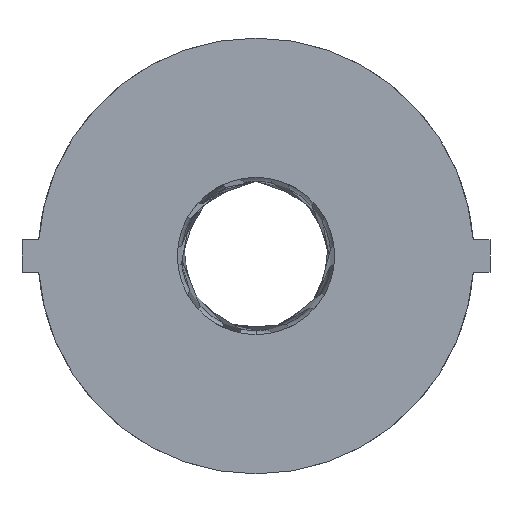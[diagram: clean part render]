
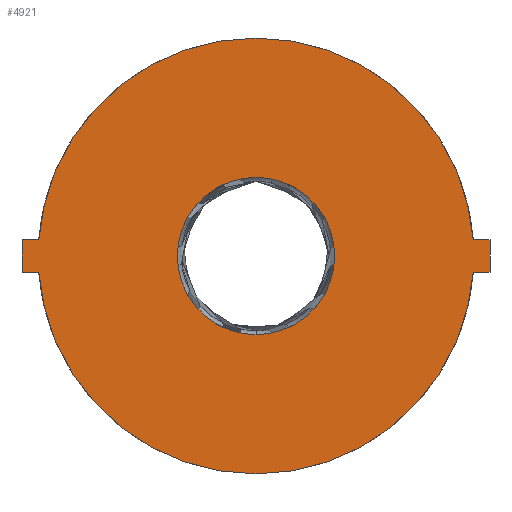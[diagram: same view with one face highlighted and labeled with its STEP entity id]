
A CAD part, front view. The second image highlights one B-rep face of the part: STEP entity #4921.
In plain terms, the highlighted planar face has unit normal (0, -1, 0).
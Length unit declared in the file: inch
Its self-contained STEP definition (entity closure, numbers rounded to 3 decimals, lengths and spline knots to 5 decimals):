
#85 = EDGE_CURVE ( 'NONE', #1512, #594, #125, .T. ) ;
#125 = CIRCLE ( 'NONE', #4471, 0.54 ) ;
#191 = ORIENTED_EDGE ( 'NONE', *, *, #5445, .T. ) ;
#195 = LINE ( 'NONE', #5136, #3071 ) ;
#203 = EDGE_CURVE ( 'NONE', #1984, #433, #4160, .T. ) ;
#219 = VECTOR ( 'NONE', #4748, 39.37008 ) ;
#260 = VERTEX_POINT ( 'NONE', #291 ) ;
#291 = CARTESIAN_POINT ( 'NONE',  ( -0.58, 0., 0.04 ) ) ;
#392 = EDGE_LOOP ( 'NONE', ( #191, #1604 ) ) ;
#433 = VERTEX_POINT ( 'NONE', #6482 ) ;
#450 = DIRECTION ( 'NONE',  ( 1., 0., 0. ) ) ;
#456 = VECTOR ( 'NONE', #450, 39.37008 ) ;
#557 = CARTESIAN_POINT ( 'NONE',  ( -0.58, 0., -0.04 ) ) ;
#594 = VERTEX_POINT ( 'NONE', #6602 ) ;
#601 = CARTESIAN_POINT ( 'NONE',  ( 0., 0., 0.54 ) ) ;
#624 = CIRCLE ( 'NONE', #6725, 0.54 ) ;
#656 = CARTESIAN_POINT ( 'NONE',  ( 0.58, 0., 0.04 ) ) ;
#1033 = ORIENTED_EDGE ( 'NONE', *, *, #3406, .T. ) ;
#1054 = CARTESIAN_POINT ( 'NONE',  ( 0., 0., 0. ) ) ;
#1084 = DIRECTION ( 'NONE',  ( -1., 0., 0. ) ) ;
#1099 = VERTEX_POINT ( 'NONE', #1756 ) ;
#1248 = DIRECTION ( 'NONE',  ( 0., 0., 1. ) ) ;
#1254 = EDGE_CURVE ( 'NONE', #4690, #3625, #2750, .T. ) ;
#1309 = CIRCLE ( 'NONE', #4706, 0.195 ) ;
#1450 = AXIS2_PLACEMENT_3D ( 'NONE', #6536, #3787, #6466 ) ;
#1512 = VERTEX_POINT ( 'NONE', #2586 ) ;
#1524 = CARTESIAN_POINT ( 'NONE',  ( 0., 0., 0.04 ) ) ;
#1604 = ORIENTED_EDGE ( 'NONE', *, *, #3862, .T. ) ;
#1605 = CARTESIAN_POINT ( 'NONE',  ( -0.58, 0., 0. ) ) ;
#1655 = CIRCLE ( 'NONE', #5702, 0.54 ) ;
#1756 = CARTESIAN_POINT ( 'NONE',  ( 0., 0., -0.195 ) ) ;
#1763 = CARTESIAN_POINT ( 'NONE',  ( -0.53852, 0., 0.04 ) ) ;
#1826 = CIRCLE ( 'NONE', #5029, 0.195 ) ;
#1984 = VERTEX_POINT ( 'NONE', #2111 ) ;
#1992 = FACE_BOUND ( 'NONE', #392, .T. ) ;
#2099 = EDGE_CURVE ( 'NONE', #433, #1512, #1655, .T. ) ;
#2111 = CARTESIAN_POINT ( 'NONE',  ( 0.58, 0., -0.04 ) ) ;
#2150 = AXIS2_PLACEMENT_3D ( 'NONE', #4991, #6590, #3428 ) ;
#2356 = ORIENTED_EDGE ( 'NONE', *, *, #6309, .T. ) ;
#2586 = CARTESIAN_POINT ( 'NONE',  ( 0., 0., -0.54 ) ) ;
#2596 = CARTESIAN_POINT ( 'NONE',  ( 0., 0., -0.04 ) ) ;
#2605 = ORIENTED_EDGE ( 'NONE', *, *, #203, .F. ) ;
#2703 = CARTESIAN_POINT ( 'NONE',  ( 0., 0., 0. ) ) ;
#2714 = VERTEX_POINT ( 'NONE', #557 ) ;
#2750 = CIRCLE ( 'NONE', #1450, 0.54 ) ;
#2804 = EDGE_CURVE ( 'NONE', #4629, #3024, #3236, .T. ) ;
#2854 = PLANE ( 'NONE',  #2150 ) ;
#3017 = ORIENTED_EDGE ( 'NONE', *, *, #2099, .F. ) ;
#3024 = VERTEX_POINT ( 'NONE', #3293 ) ;
#3071 = VECTOR ( 'NONE', #5674, 39.37008 ) ;
#3195 = ORIENTED_EDGE ( 'NONE', *, *, #4025, .F. ) ;
#3236 = LINE ( 'NONE', #5679, #4230 ) ;
#3293 = CARTESIAN_POINT ( 'NONE',  ( 0.53852, 0., 0.04 ) ) ;
#3406 = EDGE_CURVE ( 'NONE', #2714, #594, #5418, .T. ) ;
#3428 = DIRECTION ( 'NONE',  ( 0., 0., 1. ) ) ;
#3493 = DIRECTION ( 'NONE',  ( 0., 0., -1. ) ) ;
#3625 = VERTEX_POINT ( 'NONE', #601 ) ;
#3761 = DIRECTION ( 'NONE',  ( 0., 0., 1. ) ) ;
#3787 = DIRECTION ( 'NONE',  ( 0., 1., 0. ) ) ;
#3862 = EDGE_CURVE ( 'NONE', #6628, #1099, #1309, .T. ) ;
#3936 = EDGE_LOOP ( 'NONE', ( #3017, #2605, #5635, #4362, #3195, #4037, #6709, #2356, #1033, #6298 ) ) ;
#3948 = DIRECTION ( 'NONE',  ( 0., 1., 0. ) ) ;
#4025 = EDGE_CURVE ( 'NONE', #3625, #3024, #624, .T. ) ;
#4037 = ORIENTED_EDGE ( 'NONE', *, *, #1254, .F. ) ;
#4153 = FACE_OUTER_BOUND ( 'NONE', #3936, .T. ) ;
#4160 = LINE ( 'NONE', #2596, #219 ) ;
#4230 = VECTOR ( 'NONE', #1084, 39.37008 ) ;
#4264 = CARTESIAN_POINT ( 'NONE',  ( 0., 0., 0.195 ) ) ;
#4278 = CARTESIAN_POINT ( 'NONE',  ( 0., 0., 0. ) ) ;
#4303 = DIRECTION ( 'NONE',  ( 1., 0., 0. ) ) ;
#4362 = ORIENTED_EDGE ( 'NONE', *, *, #2804, .T. ) ;
#4381 = EDGE_CURVE ( 'NONE', #1984, #4629, #195, .T. ) ;
#4471 = AXIS2_PLACEMENT_3D ( 'NONE', #4278, #6336, #6893 ) ;
#4480 = DIRECTION ( 'NONE',  ( 0., 0., 1. ) ) ;
#4506 = CARTESIAN_POINT ( 'NONE',  ( 0., 0., 0. ) ) ;
#4629 = VERTEX_POINT ( 'NONE', #656 ) ;
#4690 = VERTEX_POINT ( 'NONE', #1763 ) ;
#4706 = AXIS2_PLACEMENT_3D ( 'NONE', #5340, #4844, #3761 ) ;
#4730 = VECTOR ( 'NONE', #4303, 39.37008 ) ;
#4748 = DIRECTION ( 'NONE',  ( -1., 0., 0. ) ) ;
#4844 = DIRECTION ( 'NONE',  ( 0., 1., 0. ) ) ;
#4852 = CARTESIAN_POINT ( 'NONE',  ( 0., 0., -0.04 ) ) ;
#4921 = ADVANCED_FACE ( 'NONE', ( #4153, #1992 ), #2854, .F. ) ;
#4991 = CARTESIAN_POINT ( 'NONE',  ( 0., 0., 0. ) ) ;
#5029 = AXIS2_PLACEMENT_3D ( 'NONE', #4506, #3948, #4480 ) ;
#5136 = CARTESIAN_POINT ( 'NONE',  ( 0.58, 0., 0. ) ) ;
#5340 = CARTESIAN_POINT ( 'NONE',  ( 0., 0., 0. ) ) ;
#5407 = DIRECTION ( 'NONE',  ( 0., 0., 1. ) ) ;
#5418 = LINE ( 'NONE', #4852, #4730 ) ;
#5445 = EDGE_CURVE ( 'NONE', #1099, #6628, #1826, .T. ) ;
#5534 = EDGE_CURVE ( 'NONE', #260, #4690, #6323, .T. ) ;
#5635 = ORIENTED_EDGE ( 'NONE', *, *, #4381, .T. ) ;
#5674 = DIRECTION ( 'NONE',  ( 0., 0., 1. ) ) ;
#5679 = CARTESIAN_POINT ( 'NONE',  ( 0., 0., 0.04 ) ) ;
#5702 = AXIS2_PLACEMENT_3D ( 'NONE', #1054, #6948, #1248 ) ;
#6070 = LINE ( 'NONE', #1605, #6477 ) ;
#6298 = ORIENTED_EDGE ( 'NONE', *, *, #85, .F. ) ;
#6309 = EDGE_CURVE ( 'NONE', #260, #2714, #6070, .T. ) ;
#6323 = LINE ( 'NONE', #1524, #456 ) ;
#6336 = DIRECTION ( 'NONE',  ( 0., 1., 0. ) ) ;
#6466 = DIRECTION ( 'NONE',  ( 0., 0., 1. ) ) ;
#6477 = VECTOR ( 'NONE', #3493, 39.37008 ) ;
#6482 = CARTESIAN_POINT ( 'NONE',  ( 0.53852, 0., -0.04 ) ) ;
#6536 = CARTESIAN_POINT ( 'NONE',  ( 0., 0., 0. ) ) ;
#6590 = DIRECTION ( 'NONE',  ( 0., 1., 0. ) ) ;
#6602 = CARTESIAN_POINT ( 'NONE',  ( -0.53852, 0., -0.04 ) ) ;
#6628 = VERTEX_POINT ( 'NONE', #4264 ) ;
#6709 = ORIENTED_EDGE ( 'NONE', *, *, #5534, .F. ) ;
#6725 = AXIS2_PLACEMENT_3D ( 'NONE', #2703, #6935, #5407 ) ;
#6893 = DIRECTION ( 'NONE',  ( 0., 0., 1. ) ) ;
#6935 = DIRECTION ( 'NONE',  ( 0., 1., 0. ) ) ;
#6948 = DIRECTION ( 'NONE',  ( 0., 1., 0. ) ) ;
